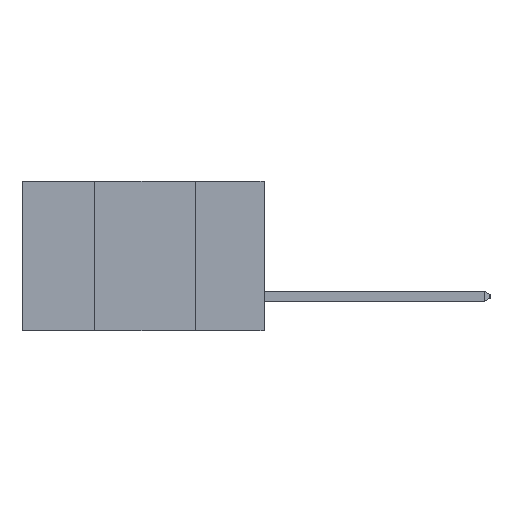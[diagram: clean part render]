
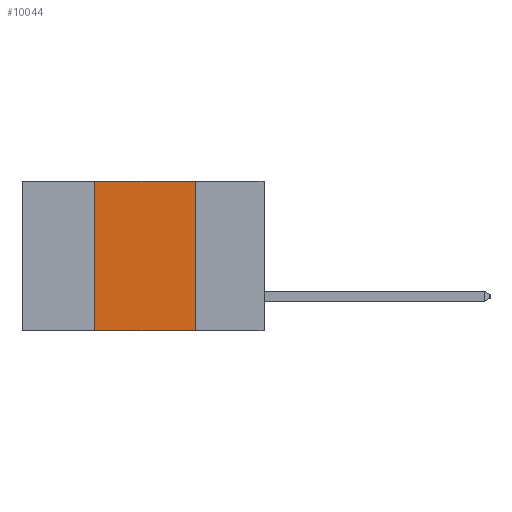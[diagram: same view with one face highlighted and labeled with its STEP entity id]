
A CAD part, left-side view. The second image highlights one B-rep face of the part: STEP entity #10044.
In plain terms, the highlighted planar face has unit normal (-1, 0, 0).
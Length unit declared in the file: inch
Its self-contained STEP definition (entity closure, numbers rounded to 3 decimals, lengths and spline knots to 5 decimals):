
#203 = DIRECTION ( 'NONE',  ( 0., -1., 0. ) ) ;
#1060 = LINE ( 'NONE', #4374, #11924 ) ;
#1640 = LINE ( 'NONE', #1826, #9336 ) ;
#1826 = CARTESIAN_POINT ( 'NONE',  ( 0., 0.6, 0. ) ) ;
#1901 = VERTEX_POINT ( 'NONE', #16858 ) ;
#1962 = LINE ( 'NONE', #18319, #10628 ) ;
#2955 = EDGE_CURVE ( 'NONE', #11159, #4944, #8672, .T. ) ;
#3028 = CARTESIAN_POINT ( 'NONE',  ( 0., 0.17, 0. ) ) ;
#3339 = PLANE ( 'NONE',  #8856 ) ;
#4374 = CARTESIAN_POINT ( 'NONE',  ( 0., 0.6, -0.37 ) ) ;
#4944 = VERTEX_POINT ( 'NONE', #8010 ) ;
#6413 = CARTESIAN_POINT ( 'NONE',  ( 0., 0.6, 0. ) ) ;
#6481 = DIRECTION ( 'NONE',  ( 0., 0., -1. ) ) ;
#7750 = FACE_OUTER_BOUND ( 'NONE', #17823, .T. ) ;
#8010 = CARTESIAN_POINT ( 'NONE',  ( 0., 0.17, -0.37 ) ) ;
#8486 = EDGE_CURVE ( 'NONE', #12586, #11159, #1640, .T. ) ;
#8672 = LINE ( 'NONE', #16374, #12280 ) ;
#8856 = AXIS2_PLACEMENT_3D ( 'NONE', #6413, #15542, #6481 ) ;
#9297 = ORIENTED_EDGE ( 'NONE', *, *, #2955, .F. ) ;
#9336 = VECTOR ( 'NONE', #203, 39.37008 ) ;
#10044 = ADVANCED_FACE ( 'NONE', ( #7750 ), #3339, .F. ) ;
#10628 = VECTOR ( 'NONE', #15299, 39.37008 ) ;
#11159 = VERTEX_POINT ( 'NONE', #3028 ) ;
#11679 = CARTESIAN_POINT ( 'NONE',  ( 0., 0.42, 0. ) ) ;
#11924 = VECTOR ( 'NONE', #15016, 39.37008 ) ;
#12280 = VECTOR ( 'NONE', #15895, 39.37008 ) ;
#12586 = VERTEX_POINT ( 'NONE', #11679 ) ;
#13191 = ORIENTED_EDGE ( 'NONE', *, *, #17375, .F. ) ;
#13354 = EDGE_CURVE ( 'NONE', #1901, #4944, #1060, .T. ) ;
#15016 = DIRECTION ( 'NONE',  ( 0., -1., 0. ) ) ;
#15299 = DIRECTION ( 'NONE',  ( 0., 0., 1. ) ) ;
#15542 = DIRECTION ( 'NONE',  ( 1., 0., 0. ) ) ;
#15895 = DIRECTION ( 'NONE',  ( 0., 0., -1. ) ) ;
#16374 = CARTESIAN_POINT ( 'NONE',  ( 0., 0.17, -0.37 ) ) ;
#16858 = CARTESIAN_POINT ( 'NONE',  ( 0., 0.42, -0.37 ) ) ;
#17375 = EDGE_CURVE ( 'NONE', #1901, #12586, #1962, .T. ) ;
#17823 = EDGE_LOOP ( 'NONE', ( #9297, #18780, #13191, #18175 ) ) ;
#18175 = ORIENTED_EDGE ( 'NONE', *, *, #13354, .T. ) ;
#18319 = CARTESIAN_POINT ( 'NONE',  ( 0., 0.42, -0.37 ) ) ;
#18780 = ORIENTED_EDGE ( 'NONE', *, *, #8486, .F. ) ;
